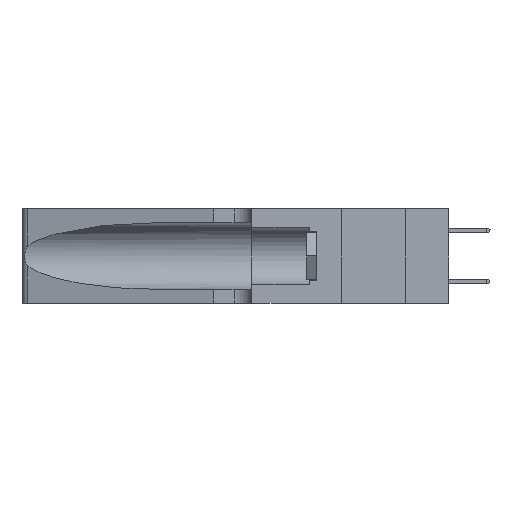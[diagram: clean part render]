
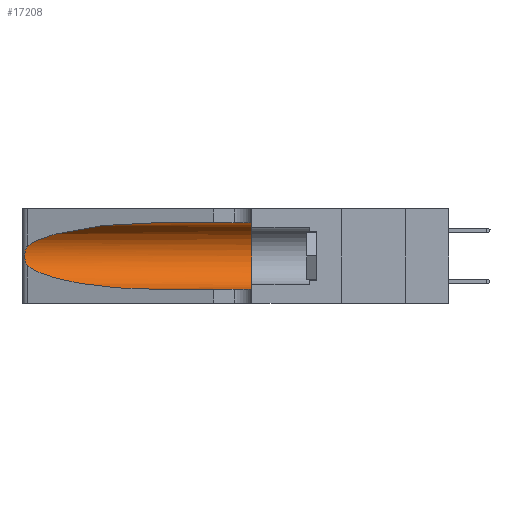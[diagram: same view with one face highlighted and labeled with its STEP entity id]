
A CAD part, left-side view. The second image highlights one B-rep face of the part: STEP entity #17208.
In plain terms, the highlighted cylindrical face has radius 3.308 mm (diameter 6.617 mm), a partial arc.
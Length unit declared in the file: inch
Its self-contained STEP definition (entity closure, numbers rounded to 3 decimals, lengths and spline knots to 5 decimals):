
#1321 = VERTEX_POINT ( 'NONE', #22104 ) ;
#1688 = VERTEX_POINT ( 'NONE', #34820 ) ;
#3302 = CARTESIAN_POINT ( 'NONE',  ( 0.1305, 0.72297, 0.31525 ) ) ;
#3482 = CARTESIAN_POINT ( 'NONE',  ( 0.25856, 1.23593, 0.16098 ) ) ;
#4105 =( BOUNDED_CURVE ( )  B_SPLINE_CURVE ( 3, ( #14808, #39989, #18493, #43575 ),
 .UNSPECIFIED., .F., .T. ) 
 B_SPLINE_CURVE_WITH_KNOTS ( ( 4, 4 ),
 ( 1.5708, 2.84003 ),
 .UNSPECIFIED. ) 
 CURVE ( )  GEOMETRIC_REPRESENTATION_ITEM ( )  RATIONAL_B_SPLINE_CURVE ( ( 1., 0.87, 0.87, 1. ) ) 
 REPRESENTATION_ITEM ( '' )  );
#4842 = EDGE_CURVE ( 'NONE', #1688, #25129, #21135, .T. ) ;
#5148 = LINE ( 'NONE', #23256, #23403 ) ;
#6486 = CARTESIAN_POINT ( 'NONE',  ( 0.1305, 1.61858, 0.185 ) ) ;
#7229 = CARTESIAN_POINT ( 'NONE',  ( 0.25639, 1.23186, 0.15144 ) ) ;
#7300 = CARTESIAN_POINT ( 'NONE',  ( 0.25487, 1.22718, 0.14631 ) ) ;
#8559 = DIRECTION ( 'NONE',  ( 0., 1., 0. ) ) ;
#8936 = AXIS2_PLACEMENT_3D ( 'NONE', #6486, #31885, #10226 ) ;
#9458 = CARTESIAN_POINT ( 'NONE',  ( 0.25487, 1.22718, 0.14631 ) ) ;
#9615 = CARTESIAN_POINT ( 'NONE',  ( 0.1305, 0.72297, 0.05475 ) ) ;
#10226 = DIRECTION ( 'NONE',  ( 0., 0., -1. ) ) ;
#10806 = CARTESIAN_POINT ( 'NONE',  ( 0.1305, 0.35, 0.05475 ) ) ;
#10946 = CARTESIAN_POINT ( 'NONE',  ( 0.25487, 1.22718, 0.14631 ) ) ;
#11307 = EDGE_CURVE ( 'NONE', #26649, #1688, #4105, .T. ) ;
#12233 = DIRECTION ( 'NONE',  ( 0., -1., 0. ) ) ;
#13784 = CARTESIAN_POINT ( 'NONE',  ( 0.25639, 1.23184, 0.21858 ) ) ;
#14808 = CARTESIAN_POINT ( 'NONE',  ( 0.1305, 0.72297, 0.31525 ) ) ;
#15167 = VERTEX_POINT ( 'NONE', #10806 ) ;
#16940 = EDGE_CURVE ( 'NONE', #41502, #15167, #5148, .T. ) ;
#17208 = ADVANCED_FACE ( 'NONE', ( #22832 ), #20584, .F. ) ;
#17471 = CARTESIAN_POINT ( 'NONE',  ( 0.25854, 1.2359, 0.20912 ) ) ;
#18493 = CARTESIAN_POINT ( 'NONE',  ( 0.2373, 1.15595, 0.28018 ) ) ;
#20092 = AXIS2_PLACEMENT_3D ( 'NONE', #30246, #8559, #33879 ) ;
#20584 = CYLINDRICAL_SURFACE ( 'NONE', #8936, 0.13025 ) ;
#20647 = EDGE_CURVE ( 'NONE', #25129, #41502, #26018, .T. ) ;
#21135 = B_SPLINE_CURVE_WITH_KNOTS ( 'NONE', 3,
 ( #28172, #24412, #13784, #38990, #17471, #42588, #21736, #46815, #25366, #3482, #28934, #7229, #32601, #10946 ),
 .UNSPECIFIED., .F., .F.,
 ( 4, 2, 2, 2, 2, 2, 4 ),
 ( 0., 0.00027, 0.00053, 0.00107, 0.0016, 0.00187, 0.00214 ),
 .UNSPECIFIED. ) ;
#21736 = CARTESIAN_POINT ( 'NONE',  ( 0.26075, 1.23896, 0.19203 ) ) ;
#22104 = CARTESIAN_POINT ( 'NONE',  ( 0.1305, 0.35, 0.31525 ) ) ;
#22832 = FACE_OUTER_BOUND ( 'NONE', #27442, .T. ) ;
#23256 = CARTESIAN_POINT ( 'NONE',  ( 0.1305, 1.61858, 0.05475 ) ) ;
#23403 = VECTOR ( 'NONE', #26886, 39.37008 ) ;
#23789 = CIRCLE ( 'NONE', #20092, 0.13025 ) ;
#24391 = ORIENTED_EDGE ( 'NONE', *, *, #11307, .T. ) ;
#24412 = CARTESIAN_POINT ( 'NONE',  ( 0.25555, 1.22994, 0.2215 ) ) ;
#25129 = VERTEX_POINT ( 'NONE', #7300 ) ;
#25366 = CARTESIAN_POINT ( 'NONE',  ( 0.26017, 1.23833, 0.17102 ) ) ;
#26018 =( BOUNDED_CURVE ( )  B_SPLINE_CURVE ( 3, ( #9458, #27675, #31306, #9615 ),
 .UNSPECIFIED., .F., .T. ) 
 B_SPLINE_CURVE_WITH_KNOTS ( ( 4, 4 ),
 ( 3.44316, 4.71239 ),
 .UNSPECIFIED. ) 
 CURVE ( )  GEOMETRIC_REPRESENTATION_ITEM ( )  RATIONAL_B_SPLINE_CURVE ( ( 1., 0.87, 0.87, 1. ) ) 
 REPRESENTATION_ITEM ( '' )  );
#26649 = VERTEX_POINT ( 'NONE', #3302 ) ;
#26886 = DIRECTION ( 'NONE',  ( 0., -1., 0. ) ) ;
#27442 = EDGE_LOOP ( 'NONE', ( #24391, #31427, #29006, #40974, #37515, #43338 ) ) ;
#27675 = CARTESIAN_POINT ( 'NONE',  ( 0.2373, 1.15595, 0.08982 ) ) ;
#28172 = CARTESIAN_POINT ( 'NONE',  ( 0.25487, 1.22718, 0.22369 ) ) ;
#28934 = CARTESIAN_POINT ( 'NONE',  ( 0.25789, 1.23486, 0.15765 ) ) ;
#29006 = ORIENTED_EDGE ( 'NONE', *, *, #20647, .T. ) ;
#29148 = VECTOR ( 'NONE', #12233, 39.37008 ) ;
#30246 = CARTESIAN_POINT ( 'NONE',  ( 0.1305, 0.35, 0.185 ) ) ;
#31306 = CARTESIAN_POINT ( 'NONE',  ( 0.18966, 0.96281, 0.05475 ) ) ;
#31427 = ORIENTED_EDGE ( 'NONE', *, *, #4842, .T. ) ;
#31885 = DIRECTION ( 'NONE',  ( 0., -1., 0. ) ) ;
#31941 = EDGE_CURVE ( 'NONE', #1321, #15167, #23789, .T. ) ;
#32601 = CARTESIAN_POINT ( 'NONE',  ( 0.25555, 1.22993, 0.14849 ) ) ;
#33879 = DIRECTION ( 'NONE',  ( 0., 0., 1. ) ) ;
#34471 = EDGE_CURVE ( 'NONE', #26649, #1321, #39840, .T. ) ;
#34820 = CARTESIAN_POINT ( 'NONE',  ( 0.25487, 1.22718, 0.22369 ) ) ;
#37515 = ORIENTED_EDGE ( 'NONE', *, *, #31941, .F. ) ;
#38990 = CARTESIAN_POINT ( 'NONE',  ( 0.25787, 1.23484, 0.2124 ) ) ;
#39840 = LINE ( 'NONE', #41034, #29148 ) ;
#39989 = CARTESIAN_POINT ( 'NONE',  ( 0.18966, 0.96281, 0.31525 ) ) ;
#40974 = ORIENTED_EDGE ( 'NONE', *, *, #16940, .T. ) ;
#41034 = CARTESIAN_POINT ( 'NONE',  ( 0.1305, 1.61858, 0.31525 ) ) ;
#41502 = VERTEX_POINT ( 'NONE', #41769 ) ;
#41769 = CARTESIAN_POINT ( 'NONE',  ( 0.1305, 0.72297, 0.05475 ) ) ;
#42588 = CARTESIAN_POINT ( 'NONE',  ( 0.26018, 1.23835, 0.19895 ) ) ;
#43338 = ORIENTED_EDGE ( 'NONE', *, *, #34471, .F. ) ;
#43575 = CARTESIAN_POINT ( 'NONE',  ( 0.25487, 1.22718, 0.22369 ) ) ;
#46815 = CARTESIAN_POINT ( 'NONE',  ( 0.26075, 1.23896, 0.178 ) ) ;
